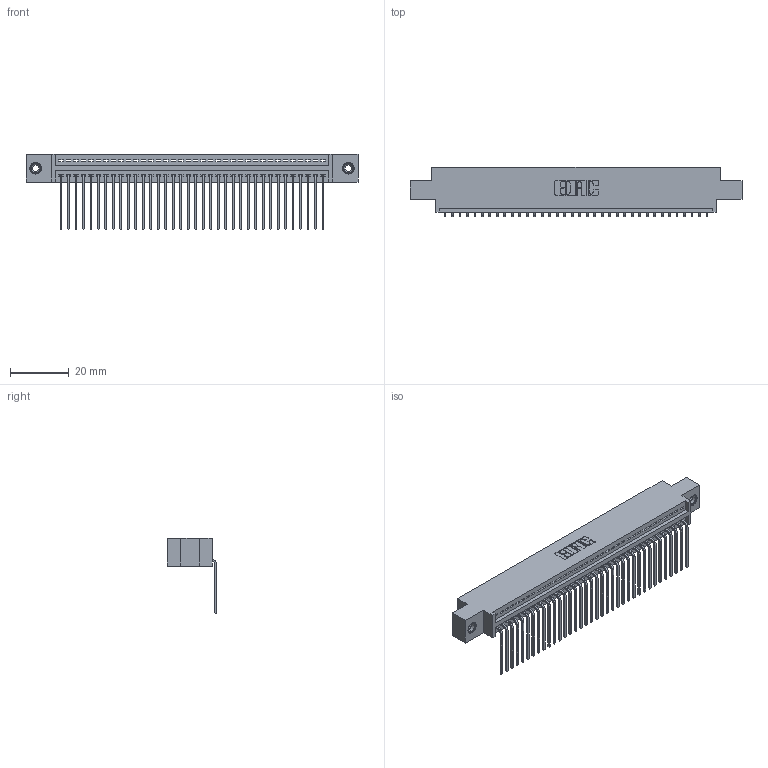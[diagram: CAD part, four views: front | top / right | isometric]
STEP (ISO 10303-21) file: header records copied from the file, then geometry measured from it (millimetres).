
FILE_DESCRIPTION (( 'STEP AP203' ), '1' );
FILE_NAME ('395-036-559-608.STEP', '2019-10-21T22:41:43', ( '' ), ( '' ), 'SwSTEP 2.0', 'SolidWorks 2016', '' );
FILE_SCHEMA (( 'CONFIG_CONTROL_DESIGN' ));
Length unit declared in the file: inch
Products named in the file (4): 345 Part_0.170 Offset - 0.156 Dia-TI; 345-250-001_345-250-003-102; 345-292-001_558 559 Tail - 1; 395-036-559-608
Assembly tree (39 placements, depth 2):
  395-036-559-608
    345 Part_0.170 Offset - 0.156 Dia-TI
    345-292-001_558 559 Tail - 1  x36
    345-250-001_345-250-003-102  x2
Bounding box: 112.65 x 16.75 x 25.53 mm (x, y, z)
Volume: 10650.4 mm3; surface area: 14922.4 mm2
Topology: 39 solids, 39 shells, 2350 faces, 7041 edges, 4638 vertices
Faces by surface type: plane 1628, cylinder 706, cone 12, torus 4
Entity records: 29304 total; most frequent: CARTESIAN_POINT 5059, ORIENTED_EDGE 5022, DIRECTION 4453, EDGE_CURVE 2511, LINE 2215, VECTOR 2215, VERTEX_POINT 1668, AXIS2_PLACEMENT_3D 1119
